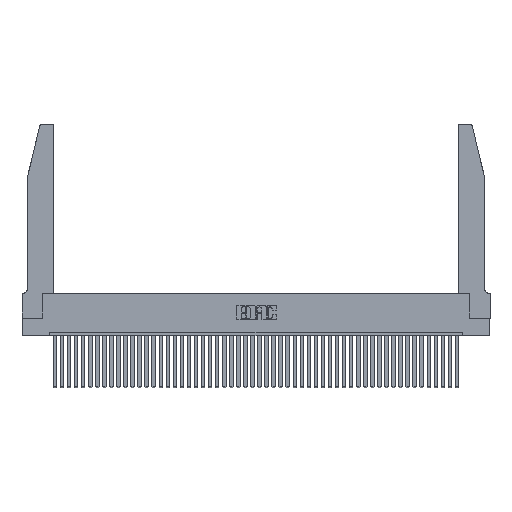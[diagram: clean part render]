
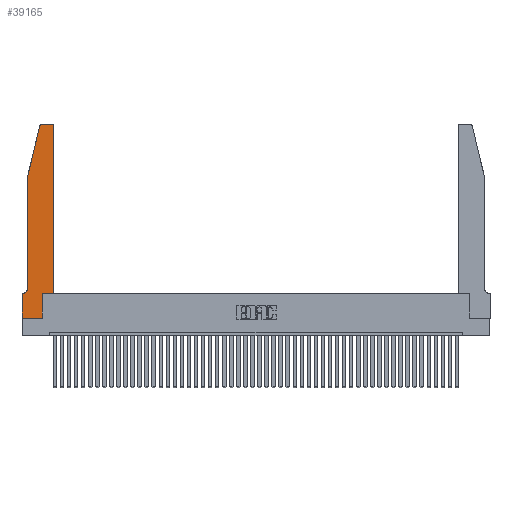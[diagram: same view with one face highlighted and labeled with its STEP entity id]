
A CAD part, top view. The second image highlights one B-rep face of the part: STEP entity #39165.
In plain terms, the highlighted planar face has unit normal (0, 0, 1).
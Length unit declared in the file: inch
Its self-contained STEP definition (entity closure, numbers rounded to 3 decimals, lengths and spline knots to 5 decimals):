
#194 = LINE ( 'NONE', #38412, #29005 ) ;
#255 = EDGE_CURVE ( 'NONE', #18523, #4474, #36267, .T. ) ;
#762 = CARTESIAN_POINT ( 'NONE',  ( 0.284, 2.72, 0.37 ) ) ;
#885 = VERTEX_POINT ( 'NONE', #38126 ) ;
#1263 = ORIENTED_EDGE ( 'NONE', *, *, #255, .T. ) ;
#2262 = DIRECTION ( 'NONE',  ( 0., -1., 0. ) ) ;
#3319 = EDGE_CURVE ( 'NONE', #45804, #12635, #17638, .T. ) ;
#3351 = CARTESIAN_POINT ( 'NONE',  ( 0., 0., 0.37 ) ) ;
#3738 = EDGE_LOOP ( 'NONE', ( #17631, #33593, #1263, #27112, #37859, #21519, #37759, #11695, #10370, #42813, #28294, #27433 ) ) ;
#3824 = VERTEX_POINT ( 'NONE', #40601 ) ;
#4394 = CARTESIAN_POINT ( 'NONE',  ( 0., 0.35, 0.37 ) ) ;
#4474 = VERTEX_POINT ( 'NONE', #5778 ) ;
#5351 = DIRECTION ( 'NONE',  ( 0., -1., 0. ) ) ;
#5778 = CARTESIAN_POINT ( 'NONE',  ( 0.0755, 2., 0.37 ) ) ;
#6272 = EDGE_CURVE ( 'NONE', #3824, #11119, #194, .T. ) ;
#6641 = VECTOR ( 'NONE', #12131, 39.37008 ) ;
#6968 = DIRECTION ( 'NONE',  ( 1., 0., 0. ) ) ;
#8150 = EDGE_CURVE ( 'NONE', #4474, #40595, #33308, .T. ) ;
#8806 = DIRECTION ( 'NONE',  ( 1., 0., 0. ) ) ;
#8999 = FACE_OUTER_BOUND ( 'NONE', #3738, .T. ) ;
#10095 = CARTESIAN_POINT ( 'NONE',  ( 0.4205, 2.72, 0.37 ) ) ;
#10370 = ORIENTED_EDGE ( 'NONE', *, *, #30199, .T. ) ;
#10858 = PLANE ( 'NONE',  #19149 ) ;
#11119 = VERTEX_POINT ( 'NONE', #32231 ) ;
#11695 = ORIENTED_EDGE ( 'NONE', *, *, #45253, .T. ) ;
#12131 = DIRECTION ( 'NONE',  ( -1., 0., 0. ) ) ;
#12607 = CARTESIAN_POINT ( 'NONE',  ( 0.0755, 0.42, 0.37 ) ) ;
#12635 = VERTEX_POINT ( 'NONE', #18635 ) ;
#12819 = CARTESIAN_POINT ( 'NONE',  ( 0.0055, 0.35, 0.37 ) ) ;
#13344 = VECTOR ( 'NONE', #29049, 39.37008 ) ;
#15845 = VECTOR ( 'NONE', #38362, 39.37008 ) ;
#16136 = DIRECTION ( 'NONE',  ( 0., 0., 1. ) ) ;
#17631 = ORIENTED_EDGE ( 'NONE', *, *, #28681, .T. ) ;
#17638 = LINE ( 'NONE', #30500, #18716 ) ;
#18195 = LINE ( 'NONE', #22267, #6641 ) ;
#18523 = VERTEX_POINT ( 'NONE', #38445 ) ;
#18635 = CARTESIAN_POINT ( 'NONE',  ( 0., 0., 0.37 ) ) ;
#18716 = VECTOR ( 'NONE', #2262, 39.37008 ) ;
#18733 = AXIS2_PLACEMENT_3D ( 'NONE', #10095, #38423, #6968 ) ;
#19149 = AXIS2_PLACEMENT_3D ( 'NONE', #4394, #21622, #29213 ) ;
#19281 = EDGE_CURVE ( 'NONE', #11119, #885, #33435, .T. ) ;
#19449 = CIRCLE ( 'NONE', #18733, 0.03 ) ;
#19547 = AXIS2_PLACEMENT_3D ( 'NONE', #762, #16136, #8806 ) ;
#19982 = VECTOR ( 'NONE', #5351, 39.37008 ) ;
#20357 = CARTESIAN_POINT ( 'NONE',  ( 0., 0.35, 0.37 ) ) ;
#21513 = VERTEX_POINT ( 'NONE', #24584 ) ;
#21519 = ORIENTED_EDGE ( 'NONE', *, *, #45459, .T. ) ;
#21622 = DIRECTION ( 'NONE',  ( 0., 0., 1. ) ) ;
#21885 = CARTESIAN_POINT ( 'NONE',  ( 0.2865, 0., 0.37 ) ) ;
#22267 = CARTESIAN_POINT ( 'NONE',  ( 0.2605, 2.75, 0.37 ) ) ;
#22865 = DIRECTION ( 'NONE',  ( -1., 0., 0. ) ) ;
#23053 = CARTESIAN_POINT ( 'NONE',  ( 0.0755, 2., 0.37 ) ) ;
#23091 = CARTESIAN_POINT ( 'NONE',  ( 0.2865, 0.35, 0.37 ) ) ;
#24584 = CARTESIAN_POINT ( 'NONE',  ( 0.4205, 2.75, 0.37 ) ) ;
#25054 = CARTESIAN_POINT ( 'NONE',  ( 0.4505, 0.35, 0.37 ) ) ;
#25469 = CARTESIAN_POINT ( 'NONE',  ( 0.0755, 0.35, 0.37 ) ) ;
#26836 = DIRECTION ( 'NONE',  ( -0.239, -0.971, 0. ) ) ;
#27112 = ORIENTED_EDGE ( 'NONE', *, *, #8150, .T. ) ;
#27433 = ORIENTED_EDGE ( 'NONE', *, *, #44877, .T. ) ;
#28294 = ORIENTED_EDGE ( 'NONE', *, *, #19281, .T. ) ;
#28323 = EDGE_CURVE ( 'NONE', #39735, #18523, #38906, .T. ) ;
#28681 = EDGE_CURVE ( 'NONE', #21513, #39735, #18195, .T. ) ;
#29005 = VECTOR ( 'NONE', #41869, 39.37008 ) ;
#29049 = DIRECTION ( 'NONE',  ( 0., 1., 0. ) ) ;
#29213 = DIRECTION ( 'NONE',  ( 1., 0., 0. ) ) ;
#29958 = LINE ( 'NONE', #25469, #38397 ) ;
#30199 = EDGE_CURVE ( 'NONE', #45378, #3824, #41006, .T. ) ;
#30500 = CARTESIAN_POINT ( 'NONE',  ( 0., 0., 0.37 ) ) ;
#30654 = DIRECTION ( 'NONE',  ( 0., 0., -1. ) ) ;
#32231 = CARTESIAN_POINT ( 'NONE',  ( 0.4505, 0.35, 0.37 ) ) ;
#32572 = EDGE_CURVE ( 'NONE', #40595, #40054, #39732, .T. ) ;
#32802 = DIRECTION ( 'NONE',  ( -1., 0., 0. ) ) ;
#33308 = LINE ( 'NONE', #23053, #19982 ) ;
#33435 = LINE ( 'NONE', #25054, #13344 ) ;
#33593 = ORIENTED_EDGE ( 'NONE', *, *, #28323, .T. ) ;
#34326 = CARTESIAN_POINT ( 'NONE',  ( 0.0755, 2., 0.37 ) ) ;
#34920 = DIRECTION ( 'NONE',  ( 1., 0., 0. ) ) ;
#35623 = LINE ( 'NONE', #3351, #43411 ) ;
#36267 = LINE ( 'NONE', #34326, #40761 ) ;
#37687 = CARTESIAN_POINT ( 'NONE',  ( 0.0055, 0.42, 0.37 ) ) ;
#37759 = ORIENTED_EDGE ( 'NONE', *, *, #3319, .T. ) ;
#37859 = ORIENTED_EDGE ( 'NONE', *, *, #32572, .T. ) ;
#38126 = CARTESIAN_POINT ( 'NONE',  ( 0.4505, 2.72, 0.37 ) ) ;
#38362 = DIRECTION ( 'NONE',  ( 0., 1., 0. ) ) ;
#38397 = VECTOR ( 'NONE', #32802, 39.37008 ) ;
#38412 = CARTESIAN_POINT ( 'NONE',  ( 0.4505, 0.35, 0.37 ) ) ;
#38423 = DIRECTION ( 'NONE',  ( 0., 0., 1. ) ) ;
#38445 = CARTESIAN_POINT ( 'NONE',  ( 0.25487, 2.72718, 0.37 ) ) ;
#38906 = CIRCLE ( 'NONE', #19547, 0.03 ) ;
#39165 = ADVANCED_FACE ( 'NONE', ( #8999 ), #10858, .T. ) ;
#39732 = CIRCLE ( 'NONE', #40589, 0.07 ) ;
#39735 = VERTEX_POINT ( 'NONE', #42811 ) ;
#40054 = VERTEX_POINT ( 'NONE', #12819 ) ;
#40589 = AXIS2_PLACEMENT_3D ( 'NONE', #37687, #30654, #22865 ) ;
#40595 = VERTEX_POINT ( 'NONE', #12607 ) ;
#40601 = CARTESIAN_POINT ( 'NONE',  ( 0.2865, 0.35, 0.37 ) ) ;
#40761 = VECTOR ( 'NONE', #26836, 39.37008 ) ;
#41006 = LINE ( 'NONE', #23091, #15845 ) ;
#41869 = DIRECTION ( 'NONE',  ( 1., 0., 0. ) ) ;
#42811 = CARTESIAN_POINT ( 'NONE',  ( 0.284, 2.75, 0.37 ) ) ;
#42813 = ORIENTED_EDGE ( 'NONE', *, *, #6272, .T. ) ;
#43411 = VECTOR ( 'NONE', #34920, 39.37008 ) ;
#44877 = EDGE_CURVE ( 'NONE', #885, #21513, #19449, .T. ) ;
#45253 = EDGE_CURVE ( 'NONE', #12635, #45378, #35623, .T. ) ;
#45378 = VERTEX_POINT ( 'NONE', #21885 ) ;
#45459 = EDGE_CURVE ( 'NONE', #40054, #45804, #29958, .T. ) ;
#45804 = VERTEX_POINT ( 'NONE', #20357 ) ;
